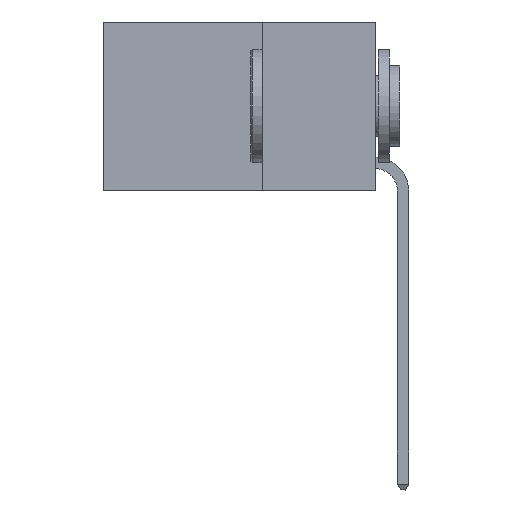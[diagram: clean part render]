
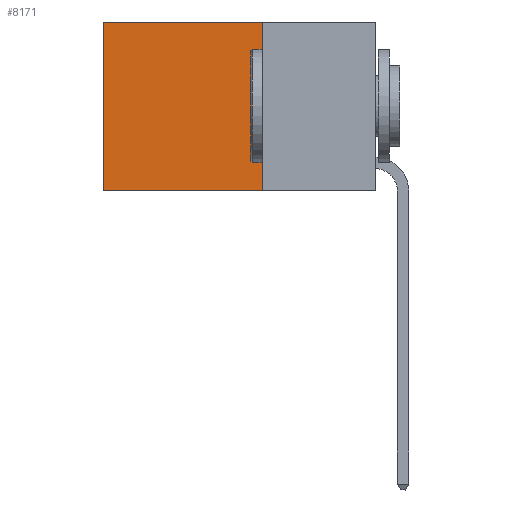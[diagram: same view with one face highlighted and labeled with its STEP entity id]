
A CAD part, left-side view. The second image highlights one B-rep face of the part: STEP entity #8171.
In plain terms, the highlighted planar face has unit normal (-1, 0, 0).
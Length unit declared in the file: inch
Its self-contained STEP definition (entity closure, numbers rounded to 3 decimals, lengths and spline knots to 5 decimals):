
#335 = VECTOR ( 'NONE', #6427, 39.37008 ) ;
#1117 = ORIENTED_EDGE ( 'NONE', *, *, #9221, .F. ) ;
#1373 = VERTEX_POINT ( 'NONE', #11535 ) ;
#2070 = ORIENTED_EDGE ( 'NONE', *, *, #3413, .T. ) ;
#2477 = CARTESIAN_POINT ( 'NONE',  ( 0.2625, 0.6, 0. ) ) ;
#2919 = DIRECTION ( 'NONE',  ( 0., 0., -1. ) ) ;
#3399 = EDGE_CURVE ( 'NONE', #10016, #3488, #14379, .T. ) ;
#3413 = EDGE_CURVE ( 'NONE', #3488, #1373, #13572, .T. ) ;
#3488 = VERTEX_POINT ( 'NONE', #10587 ) ;
#3900 = CARTESIAN_POINT ( 'NONE',  ( 0.2625, 0.25, -0.37 ) ) ;
#4045 = DIRECTION ( 'NONE',  ( 0., 1., 0. ) ) ;
#4048 = VECTOR ( 'NONE', #5398, 39.37008 ) ;
#4089 = CARTESIAN_POINT ( 'NONE',  ( 0.2625, 0.25, 0. ) ) ;
#4192 = CARTESIAN_POINT ( 'NONE',  ( 0.2625, 0.25, 0. ) ) ;
#4450 = LINE ( 'NONE', #4089, #4048 ) ;
#5085 = CARTESIAN_POINT ( 'NONE',  ( 0.2625, 0.25, 0. ) ) ;
#5255 = ORIENTED_EDGE ( 'NONE', *, *, #5474, .F. ) ;
#5398 = DIRECTION ( 'NONE',  ( 0., 0., -1. ) ) ;
#5474 = EDGE_CURVE ( 'NONE', #14641, #1373, #13700, .T. ) ;
#6178 = ORIENTED_EDGE ( 'NONE', *, *, #3399, .T. ) ;
#6258 = AXIS2_PLACEMENT_3D ( 'NONE', #4192, #10835, #2919 ) ;
#6427 = DIRECTION ( 'NONE',  ( 0., 0., -1. ) ) ;
#7955 = CARTESIAN_POINT ( 'NONE',  ( 0.2625, 0.25, -0.37 ) ) ;
#8171 = ADVANCED_FACE ( 'NONE', ( #13540 ), #8217, .F. ) ;
#8217 = PLANE ( 'NONE',  #6258 ) ;
#9221 = EDGE_CURVE ( 'NONE', #10016, #14641, #4450, .T. ) ;
#9243 = EDGE_LOOP ( 'NONE', ( #2070, #5255, #1117, #6178 ) ) ;
#10016 = VERTEX_POINT ( 'NONE', #10866 ) ;
#10532 = VECTOR ( 'NONE', #15605, 39.37008 ) ;
#10587 = CARTESIAN_POINT ( 'NONE',  ( 0.2625, 0.6, 0. ) ) ;
#10835 = DIRECTION ( 'NONE',  ( 1., 0., 0. ) ) ;
#10866 = CARTESIAN_POINT ( 'NONE',  ( 0.2625, 0.25, 0. ) ) ;
#11535 = CARTESIAN_POINT ( 'NONE',  ( 0.2625, 0.6, -0.37 ) ) ;
#13540 = FACE_OUTER_BOUND ( 'NONE', #9243, .T. ) ;
#13572 = LINE ( 'NONE', #2477, #335 ) ;
#13700 = LINE ( 'NONE', #7955, #16364 ) ;
#14379 = LINE ( 'NONE', #5085, #10532 ) ;
#14641 = VERTEX_POINT ( 'NONE', #3900 ) ;
#15605 = DIRECTION ( 'NONE',  ( 0., 1., 0. ) ) ;
#16364 = VECTOR ( 'NONE', #4045, 39.37008 ) ;
